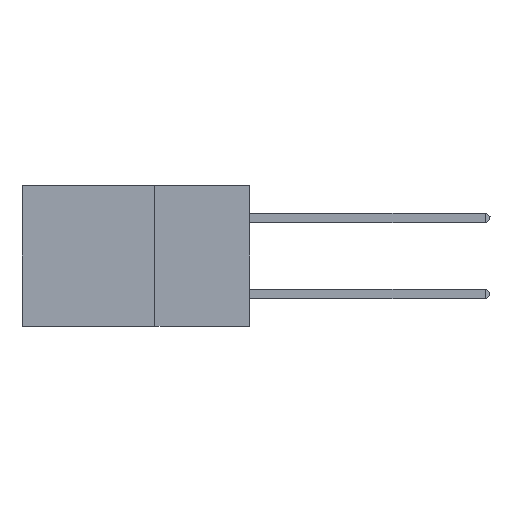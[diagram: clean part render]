
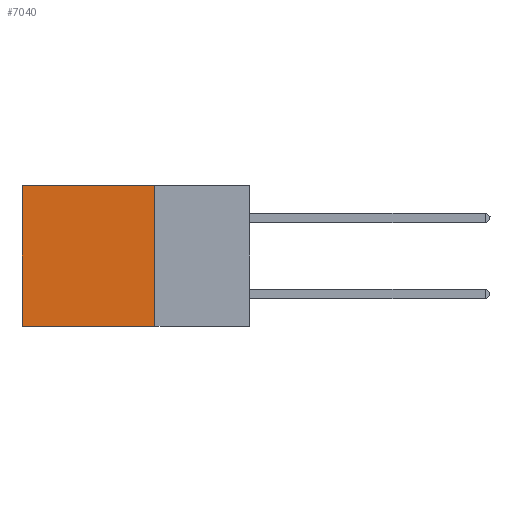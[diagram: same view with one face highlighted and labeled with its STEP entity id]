
A CAD part, left-side view. The second image highlights one B-rep face of the part: STEP entity #7040.
In plain terms, the highlighted planar face has unit normal (-1, 0, 0).
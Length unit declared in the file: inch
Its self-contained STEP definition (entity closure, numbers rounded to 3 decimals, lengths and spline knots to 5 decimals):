
#531 = VERTEX_POINT ( 'NONE', #5795 ) ;
#832 = DIRECTION ( 'NONE',  ( 0., 0., -1. ) ) ;
#2501 = CARTESIAN_POINT ( 'NONE',  ( 0.2875, 0.6, 0. ) ) ;
#3449 = ORIENTED_EDGE ( 'NONE', *, *, #17486, .T. ) ;
#5795 = CARTESIAN_POINT ( 'NONE',  ( 0.2875, 0.25, -0.37 ) ) ;
#7040 = ADVANCED_FACE ( 'NONE', ( #28419 ), #42565, .F. ) ;
#7452 = CARTESIAN_POINT ( 'NONE',  ( 0.2875, 0.25, 0. ) ) ;
#7766 = LINE ( 'NONE', #25347, #28519 ) ;
#9905 = VERTEX_POINT ( 'NONE', #25928 ) ;
#13965 = DIRECTION ( 'NONE',  ( 0., 0., -1. ) ) ;
#14041 = CARTESIAN_POINT ( 'NONE',  ( 0.2875, 0.25, -0.37 ) ) ;
#17486 = EDGE_CURVE ( 'NONE', #32936, #30012, #7766, .T. ) ;
#17567 = ORIENTED_EDGE ( 'NONE', *, *, #37845, .F. ) ;
#18156 = DIRECTION ( 'NONE',  ( 0., 0., -1. ) ) ;
#18220 = CARTESIAN_POINT ( 'NONE',  ( 0.2875, 0.25, 0. ) ) ;
#20811 = AXIS2_PLACEMENT_3D ( 'NONE', #18220, #32565, #832 ) ;
#21189 = DIRECTION ( 'NONE',  ( 0., 1., 0. ) ) ;
#25347 = CARTESIAN_POINT ( 'NONE',  ( 0.2875, 0.25, 0. ) ) ;
#25928 = CARTESIAN_POINT ( 'NONE',  ( 0.2875, 0.6, -0.37 ) ) ;
#26661 = CARTESIAN_POINT ( 'NONE',  ( 0.2875, 0.6, 0. ) ) ;
#27445 = EDGE_LOOP ( 'NONE', ( #40273, #40114, #17567, #3449 ) ) ;
#28419 = FACE_OUTER_BOUND ( 'NONE', #27445, .T. ) ;
#28519 = VECTOR ( 'NONE', #32528, 39.37008 ) ;
#30012 = VERTEX_POINT ( 'NONE', #26661 ) ;
#30708 = CARTESIAN_POINT ( 'NONE',  ( 0.2875, 0.25, 0. ) ) ;
#32528 = DIRECTION ( 'NONE',  ( 0., 1., 0. ) ) ;
#32565 = DIRECTION ( 'NONE',  ( 1., 0., 0. ) ) ;
#32936 = VERTEX_POINT ( 'NONE', #30708 ) ;
#35078 = LINE ( 'NONE', #2501, #37835 ) ;
#35107 = LINE ( 'NONE', #14041, #42074 ) ;
#37441 = EDGE_CURVE ( 'NONE', #30012, #9905, #35078, .T. ) ;
#37835 = VECTOR ( 'NONE', #18156, 39.37008 ) ;
#37845 = EDGE_CURVE ( 'NONE', #32936, #531, #38489, .T. ) ;
#38489 = LINE ( 'NONE', #7452, #43333 ) ;
#40114 = ORIENTED_EDGE ( 'NONE', *, *, #43253, .F. ) ;
#40273 = ORIENTED_EDGE ( 'NONE', *, *, #37441, .T. ) ;
#42074 = VECTOR ( 'NONE', #21189, 39.37008 ) ;
#42565 = PLANE ( 'NONE',  #20811 ) ;
#43253 = EDGE_CURVE ( 'NONE', #531, #9905, #35107, .T. ) ;
#43333 = VECTOR ( 'NONE', #13965, 39.37008 ) ;
